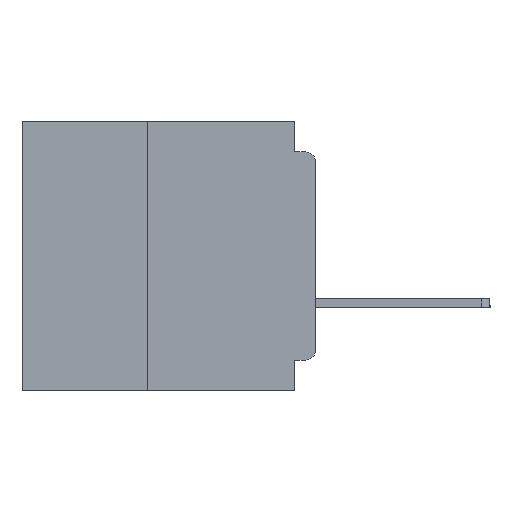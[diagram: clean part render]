
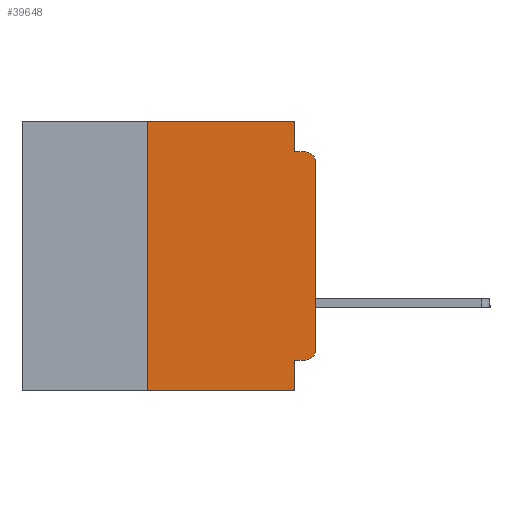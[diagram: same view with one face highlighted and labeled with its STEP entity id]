
A CAD part, left-side view. The second image highlights one B-rep face of the part: STEP entity #39648.
In plain terms, the highlighted planar face has unit normal (-1, 0, 0).
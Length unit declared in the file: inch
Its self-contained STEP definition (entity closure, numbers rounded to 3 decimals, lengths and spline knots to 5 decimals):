
#887 = VERTEX_POINT ( 'NONE', #28492 ) ;
#1698 = AXIS2_PLACEMENT_3D ( 'NONE', #24415, #52532, #28497 ) ;
#2057 = DIRECTION ( 'NONE',  ( 0., 0., 1. ) ) ;
#2139 = EDGE_CURVE ( 'NONE', #42090, #29543, #44540, .T. ) ;
#2396 = DIRECTION ( 'NONE',  ( 0., 0., -1. ) ) ;
#2552 = CIRCLE ( 'NONE', #1698, 0.015 ) ;
#2640 = AXIS2_PLACEMENT_3D ( 'NONE', #14321, #42852, #18513 ) ;
#2965 = EDGE_CURVE ( 'NONE', #29543, #29460, #28030, .T. ) ;
#3477 = CARTESIAN_POINT ( 'NONE',  ( 0., 0.031, -0.4 ) ) ;
#4156 = CARTESIAN_POINT ( 'NONE',  ( 0., 0., -0.355 ) ) ;
#4744 = EDGE_CURVE ( 'NONE', #51246, #32838, #30604, .T. ) ;
#5613 = EDGE_CURVE ( 'NONE', #42090, #42625, #51859, .T. ) ;
#6115 = VECTOR ( 'NONE', #20431, 39.37008 ) ;
#6403 = ORIENTED_EDGE ( 'NONE', *, *, #2965, .T. ) ;
#7003 = CARTESIAN_POINT ( 'NONE',  ( 0., 0., -0.34 ) ) ;
#7107 = CARTESIAN_POINT ( 'NONE',  ( 0., 0.437, -0.4 ) ) ;
#8106 = AXIS2_PLACEMENT_3D ( 'NONE', #18499, #27086, #2396 ) ;
#8819 = EDGE_CURVE ( 'NONE', #887, #42204, #37161, .T. ) ;
#10113 = ORIENTED_EDGE ( 'NONE', *, *, #39781, .F. ) ;
#11236 = DIRECTION ( 'NONE',  ( 0., -1., 0. ) ) ;
#12361 = ORIENTED_EDGE ( 'NONE', *, *, #4744, .F. ) ;
#13929 = CARTESIAN_POINT ( 'NONE',  ( 0., 0.031, 0. ) ) ;
#14081 = VECTOR ( 'NONE', #28237, 39.37008 ) ;
#14321 = CARTESIAN_POINT ( 'NONE',  ( 0., 0.015, -0.34 ) ) ;
#14340 = LINE ( 'NONE', #50048, #34865 ) ;
#16256 = CARTESIAN_POINT ( 'NONE',  ( 0., 0., 0. ) ) ;
#18499 = CARTESIAN_POINT ( 'NONE',  ( 0., 0.437, 0. ) ) ;
#18513 = DIRECTION ( 'NONE',  ( 0., 0., -1. ) ) ;
#18550 = CARTESIAN_POINT ( 'NONE',  ( 0., 0.031, -0.355 ) ) ;
#19485 = ORIENTED_EDGE ( 'NONE', *, *, #5613, .F. ) ;
#19956 = ORIENTED_EDGE ( 'NONE', *, *, #41873, .F. ) ;
#20431 = DIRECTION ( 'NONE',  ( 0., 0., 1. ) ) ;
#20528 = EDGE_CURVE ( 'NONE', #29460, #42204, #2552, .T. ) ;
#21931 = EDGE_LOOP ( 'NONE', ( #6403, #27111, #50851, #24975, #19956, #12361, #38027, #10113, #19485, #32519 ) ) ;
#22435 = DIRECTION ( 'NONE',  ( 0., 0., -1. ) ) ;
#23004 = PLANE ( 'NONE',  #8106 ) ;
#23522 = CARTESIAN_POINT ( 'NONE',  ( 0., 0.25, -0.4 ) ) ;
#24160 = CARTESIAN_POINT ( 'NONE',  ( 0., 0., -0.045 ) ) ;
#24415 = CARTESIAN_POINT ( 'NONE',  ( 0., 0.015, -0.06 ) ) ;
#24690 = VECTOR ( 'NONE', #22435, 39.37008 ) ;
#24864 = LINE ( 'NONE', #3477, #43850 ) ;
#24975 = ORIENTED_EDGE ( 'NONE', *, *, #51113, .F. ) ;
#25970 = DIRECTION ( 'NONE',  ( 0., -1., 0. ) ) ;
#27086 = DIRECTION ( 'NONE',  ( 1., 0., 0. ) ) ;
#27111 = ORIENTED_EDGE ( 'NONE', *, *, #20528, .T. ) ;
#28030 = LINE ( 'NONE', #16256, #6115 ) ;
#28142 = DIRECTION ( 'NONE',  ( 0., 0., -1. ) ) ;
#28237 = DIRECTION ( 'NONE',  ( 0., -1., 0. ) ) ;
#28492 = CARTESIAN_POINT ( 'NONE',  ( 0., 0.031, -0.045 ) ) ;
#28497 = DIRECTION ( 'NONE',  ( 0., 0., -1. ) ) ;
#28817 = DIRECTION ( 'NONE',  ( 0., 1., 0. ) ) ;
#29460 = VERTEX_POINT ( 'NONE', #30148 ) ;
#29543 = VERTEX_POINT ( 'NONE', #7003 ) ;
#30148 = CARTESIAN_POINT ( 'NONE',  ( 0., 0., -0.06 ) ) ;
#30604 = LINE ( 'NONE', #50837, #40140 ) ;
#32507 = LINE ( 'NONE', #7107, #52539 ) ;
#32519 = ORIENTED_EDGE ( 'NONE', *, *, #2139, .T. ) ;
#32838 = VERTEX_POINT ( 'NONE', #48260 ) ;
#33328 = EDGE_CURVE ( 'NONE', #51246, #37235, #32507, .T. ) ;
#34865 = VECTOR ( 'NONE', #25970, 39.37008 ) ;
#36263 = CARTESIAN_POINT ( 'NONE',  ( 0., 0.015, -0.045 ) ) ;
#36788 = LINE ( 'NONE', #13929, #24690 ) ;
#37161 = LINE ( 'NONE', #24160, #14081 ) ;
#37235 = VERTEX_POINT ( 'NONE', #52722 ) ;
#38027 = ORIENTED_EDGE ( 'NONE', *, *, #33328, .T. ) ;
#38096 = VERTEX_POINT ( 'NONE', #43101 ) ;
#39648 = ADVANCED_FACE ( 'NONE', ( #40735 ), #23004, .F. ) ;
#39781 = EDGE_CURVE ( 'NONE', #42625, #37235, #24864, .T. ) ;
#40140 = VECTOR ( 'NONE', #2057, 39.37008 ) ;
#40735 = FACE_OUTER_BOUND ( 'NONE', #21931, .T. ) ;
#41873 = EDGE_CURVE ( 'NONE', #32838, #38096, #14340, .T. ) ;
#42090 = VERTEX_POINT ( 'NONE', #43469 ) ;
#42204 = VERTEX_POINT ( 'NONE', #36263 ) ;
#42518 = VECTOR ( 'NONE', #28817, 39.37008 ) ;
#42625 = VERTEX_POINT ( 'NONE', #18550 ) ;
#42852 = DIRECTION ( 'NONE',  ( -1., 0., 0. ) ) ;
#43101 = CARTESIAN_POINT ( 'NONE',  ( 0., 0.031, 0. ) ) ;
#43469 = CARTESIAN_POINT ( 'NONE',  ( 0., 0.015, -0.355 ) ) ;
#43850 = VECTOR ( 'NONE', #28142, 39.37008 ) ;
#44540 = CIRCLE ( 'NONE', #2640, 0.015 ) ;
#48260 = CARTESIAN_POINT ( 'NONE',  ( 0., 0.25, 0. ) ) ;
#50048 = CARTESIAN_POINT ( 'NONE',  ( 0., 0.437, 0. ) ) ;
#50837 = CARTESIAN_POINT ( 'NONE',  ( 0., 0.25, -0.4 ) ) ;
#50851 = ORIENTED_EDGE ( 'NONE', *, *, #8819, .F. ) ;
#51113 = EDGE_CURVE ( 'NONE', #38096, #887, #36788, .T. ) ;
#51246 = VERTEX_POINT ( 'NONE', #23522 ) ;
#51859 = LINE ( 'NONE', #4156, #42518 ) ;
#52532 = DIRECTION ( 'NONE',  ( -1., 0., 0. ) ) ;
#52539 = VECTOR ( 'NONE', #11236, 39.37008 ) ;
#52722 = CARTESIAN_POINT ( 'NONE',  ( 0., 0.031, -0.4 ) ) ;
